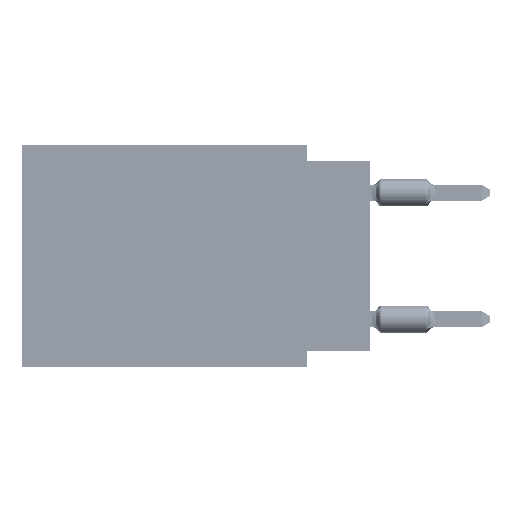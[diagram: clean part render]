
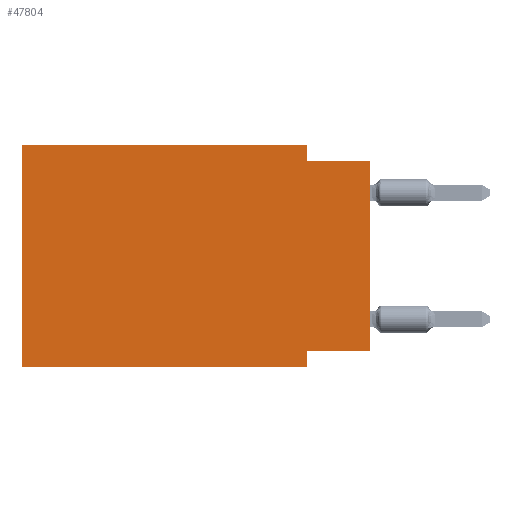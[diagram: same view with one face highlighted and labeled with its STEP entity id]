
A CAD part, left-side view. The second image highlights one B-rep face of the part: STEP entity #47804.
In plain terms, the highlighted planar face has unit normal (-1, 0, 0).
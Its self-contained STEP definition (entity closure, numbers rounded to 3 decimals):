
#425 = CARTESIAN_POINT ( 'NONE',  ( 0., 13.97, 0. ) ) ;
#1122 = EDGE_CURVE ( 'NONE', #41652, #28626, #69426, .T. ) ;
#1465 = LINE ( 'NONE', #46023, #62217 ) ;
#2633 = CARTESIAN_POINT ( 'NONE',  ( 0., 0., -8.255 ) ) ;
#2993 = LINE ( 'NONE', #2633, #11904 ) ;
#3354 = DIRECTION ( 'NONE',  ( 0., 1., 0. ) ) ;
#5932 = DIRECTION ( 'NONE',  ( 0., 0., -1. ) ) ;
#7315 = DIRECTION ( 'NONE',  ( 0., -1., 0. ) ) ;
#8395 = DIRECTION ( 'NONE',  ( 0., 0., -1. ) ) ;
#9862 = DIRECTION ( 'NONE',  ( 0., 0., 1. ) ) ;
#10724 = ORIENTED_EDGE ( 'NONE', *, *, #13610, .F. ) ;
#11904 = VECTOR ( 'NONE', #3354, 1000. ) ;
#13073 = LINE ( 'NONE', #35359, #25994 ) ;
#13610 = EDGE_CURVE ( 'NONE', #52895, #41652, #2993, .T. ) ;
#14164 = VERTEX_POINT ( 'NONE', #44151 ) ;
#14491 = EDGE_CURVE ( 'NONE', #37389, #22632, #13073, .T. ) ;
#15612 = ORIENTED_EDGE ( 'NONE', *, *, #63330, .F. ) ;
#16891 = LINE ( 'NONE', #55979, #60153 ) ;
#18714 = VERTEX_POINT ( 'NONE', #71423 ) ;
#20456 = CARTESIAN_POINT ( 'NONE',  ( 0., 13.97, 0. ) ) ;
#21901 = LINE ( 'NONE', #28105, #32535 ) ;
#22590 = CARTESIAN_POINT ( 'NONE',  ( 0., 2.54, -8.89 ) ) ;
#22632 = VERTEX_POINT ( 'NONE', #22727 ) ;
#22650 = VECTOR ( 'NONE', #8395, 1000. ) ;
#22727 = CARTESIAN_POINT ( 'NONE',  ( 0., 0., -0.635 ) ) ;
#25994 = VECTOR ( 'NONE', #57637, 1000. ) ;
#28105 = CARTESIAN_POINT ( 'NONE',  ( 0., 13.97, -8.89 ) ) ;
#28626 = VERTEX_POINT ( 'NONE', #22590 ) ;
#28714 = VERTEX_POINT ( 'NONE', #44131 ) ;
#29744 = EDGE_CURVE ( 'NONE', #28714, #14164, #1465, .T. ) ;
#31050 = CARTESIAN_POINT ( 'NONE',  ( 0., 2.54, -8.89 ) ) ;
#31309 = ORIENTED_EDGE ( 'NONE', *, *, #29744, .F. ) ;
#32535 = VECTOR ( 'NONE', #34296, 1000. ) ;
#33677 = DIRECTION ( 'NONE',  ( 0., 0., -1. ) ) ;
#34296 = DIRECTION ( 'NONE',  ( 0., -1., 0. ) ) ;
#34753 = FACE_OUTER_BOUND ( 'NONE', #65365, .T. ) ;
#35359 = CARTESIAN_POINT ( 'NONE',  ( 0., 0., -0.635 ) ) ;
#36696 = CARTESIAN_POINT ( 'NONE',  ( 0., 0., 0. ) ) ;
#37389 = VERTEX_POINT ( 'NONE', #46702 ) ;
#38698 = LINE ( 'NONE', #20456, #58162 ) ;
#41199 = EDGE_CURVE ( 'NONE', #52895, #22632, #71034, .T. ) ;
#41652 = VERTEX_POINT ( 'NONE', #69872 ) ;
#42925 = ORIENTED_EDGE ( 'NONE', *, *, #1122, .F. ) ;
#44076 = EDGE_CURVE ( 'NONE', #18714, #28626, #21901, .T. ) ;
#44131 = CARTESIAN_POINT ( 'NONE',  ( 0., 13.97, 0. ) ) ;
#44151 = CARTESIAN_POINT ( 'NONE',  ( 0., 2.54, 0. ) ) ;
#46023 = CARTESIAN_POINT ( 'NONE',  ( 0., 13.97, 0. ) ) ;
#46056 = DIRECTION ( 'NONE',  ( 1., 0., 0. ) ) ;
#46193 = ORIENTED_EDGE ( 'NONE', *, *, #50870, .F. ) ;
#46702 = CARTESIAN_POINT ( 'NONE',  ( 0., 2.54, -0.635 ) ) ;
#47032 = AXIS2_PLACEMENT_3D ( 'NONE', #425, #46056, #33677 ) ;
#47804 = ADVANCED_FACE ( 'NONE', ( #34753 ), #50475, .F. ) ;
#47870 = ORIENTED_EDGE ( 'NONE', *, *, #14491, .F. ) ;
#49536 = ORIENTED_EDGE ( 'NONE', *, *, #44076, .T. ) ;
#50475 = PLANE ( 'NONE',  #47032 ) ;
#50870 = EDGE_CURVE ( 'NONE', #14164, #37389, #16891, .T. ) ;
#52895 = VERTEX_POINT ( 'NONE', #62446 ) ;
#55524 = VECTOR ( 'NONE', #70305, 1000. ) ;
#55979 = CARTESIAN_POINT ( 'NONE',  ( 0., 2.54, 0. ) ) ;
#57637 = DIRECTION ( 'NONE',  ( 0., -1., 0. ) ) ;
#58162 = VECTOR ( 'NONE', #9862, 1000. ) ;
#60153 = VECTOR ( 'NONE', #5932, 1000. ) ;
#62217 = VECTOR ( 'NONE', #7315, 1000. ) ;
#62446 = CARTESIAN_POINT ( 'NONE',  ( 0., 0., -8.255 ) ) ;
#63330 = EDGE_CURVE ( 'NONE', #18714, #28714, #38698, .T. ) ;
#65365 = EDGE_LOOP ( 'NONE', ( #72115, #47870, #46193, #31309, #15612, #49536, #42925, #10724 ) ) ;
#69426 = LINE ( 'NONE', #31050, #22650 ) ;
#69872 = CARTESIAN_POINT ( 'NONE',  ( 0., 2.54, -8.255 ) ) ;
#70305 = DIRECTION ( 'NONE',  ( 0., 0., 1. ) ) ;
#71034 = LINE ( 'NONE', #36696, #55524 ) ;
#71423 = CARTESIAN_POINT ( 'NONE',  ( 0., 13.97, -8.89 ) ) ;
#72115 = ORIENTED_EDGE ( 'NONE', *, *, #41199, .T. ) ;
